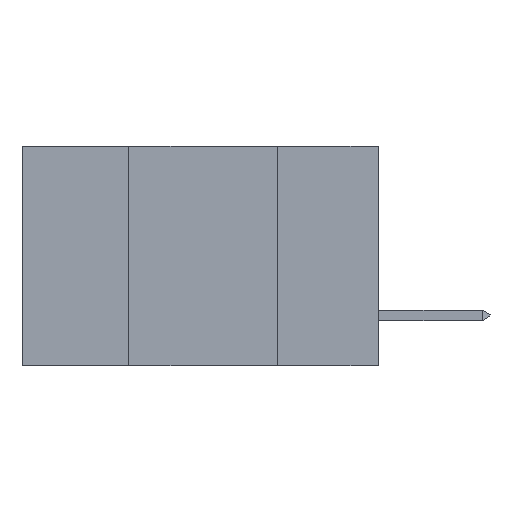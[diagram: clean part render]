
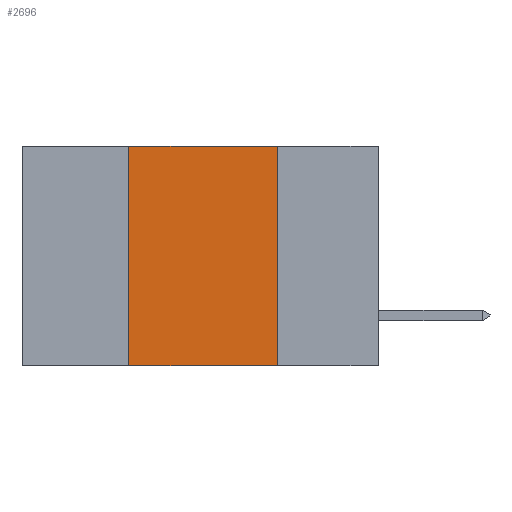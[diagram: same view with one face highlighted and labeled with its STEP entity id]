
A CAD part, left-side view. The second image highlights one B-rep face of the part: STEP entity #2696.
In plain terms, the highlighted planar face has unit normal (-1, 0, 0).
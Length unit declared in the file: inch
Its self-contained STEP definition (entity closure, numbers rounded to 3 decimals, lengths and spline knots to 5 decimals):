
#385 = EDGE_CURVE ( 'NONE', #745, #16709, #11018, .T. ) ;
#710 = CARTESIAN_POINT ( 'NONE',  ( 0., 0.6, -0.37 ) ) ;
#745 = VERTEX_POINT ( 'NONE', #5069 ) ;
#878 = DIRECTION ( 'NONE',  ( 0., -1., 0. ) ) ;
#1296 = DIRECTION ( 'NONE',  ( 1., 0., 0. ) ) ;
#2430 = AXIS2_PLACEMENT_3D ( 'NONE', #4110, #1296, #6681 ) ;
#2696 = ADVANCED_FACE ( 'NONE', ( #15519 ), #17298, .F. ) ;
#2712 = ORIENTED_EDGE ( 'NONE', *, *, #5621, .T. ) ;
#3753 = VERTEX_POINT ( 'NONE', #14832 ) ;
#3864 = EDGE_LOOP ( 'NONE', ( #13981, #5370, #6013, #2712 ) ) ;
#4032 = LINE ( 'NONE', #11311, #12004 ) ;
#4110 = CARTESIAN_POINT ( 'NONE',  ( 0., 0.6, 0. ) ) ;
#4734 = VECTOR ( 'NONE', #6929, 39.37008 ) ;
#4950 = VECTOR ( 'NONE', #9212, 39.37008 ) ;
#5069 = CARTESIAN_POINT ( 'NONE',  ( 0., 0.42, -0.37 ) ) ;
#5370 = ORIENTED_EDGE ( 'NONE', *, *, #12732, .F. ) ;
#5621 = EDGE_CURVE ( 'NONE', #745, #15732, #15391, .T. ) ;
#5797 = LINE ( 'NONE', #12248, #4734 ) ;
#6013 = ORIENTED_EDGE ( 'NONE', *, *, #385, .F. ) ;
#6290 = CARTESIAN_POINT ( 'NONE',  ( 0., 0.42, 0. ) ) ;
#6681 = DIRECTION ( 'NONE',  ( 0., 0., -1. ) ) ;
#6929 = DIRECTION ( 'NONE',  ( 0., 0., -1. ) ) ;
#9212 = DIRECTION ( 'NONE',  ( 0., 0., 1. ) ) ;
#10227 = EDGE_CURVE ( 'NONE', #3753, #15732, #5797, .T. ) ;
#11013 = VECTOR ( 'NONE', #878, 39.37008 ) ;
#11018 = LINE ( 'NONE', #6290, #4950 ) ;
#11311 = CARTESIAN_POINT ( 'NONE',  ( 0., 0.6, 0. ) ) ;
#12004 = VECTOR ( 'NONE', #15182, 39.37008 ) ;
#12248 = CARTESIAN_POINT ( 'NONE',  ( 0., 0.17, 0. ) ) ;
#12732 = EDGE_CURVE ( 'NONE', #16709, #3753, #4032, .T. ) ;
#13981 = ORIENTED_EDGE ( 'NONE', *, *, #10227, .F. ) ;
#14832 = CARTESIAN_POINT ( 'NONE',  ( 0., 0.17, 0. ) ) ;
#15182 = DIRECTION ( 'NONE',  ( 0., -1., 0. ) ) ;
#15308 = CARTESIAN_POINT ( 'NONE',  ( 0., 0.42, 0. ) ) ;
#15391 = LINE ( 'NONE', #710, #11013 ) ;
#15519 = FACE_OUTER_BOUND ( 'NONE', #3864, .T. ) ;
#15732 = VERTEX_POINT ( 'NONE', #16446 ) ;
#16446 = CARTESIAN_POINT ( 'NONE',  ( 0., 0.17, -0.37 ) ) ;
#16709 = VERTEX_POINT ( 'NONE', #15308 ) ;
#17298 = PLANE ( 'NONE',  #2430 ) ;
